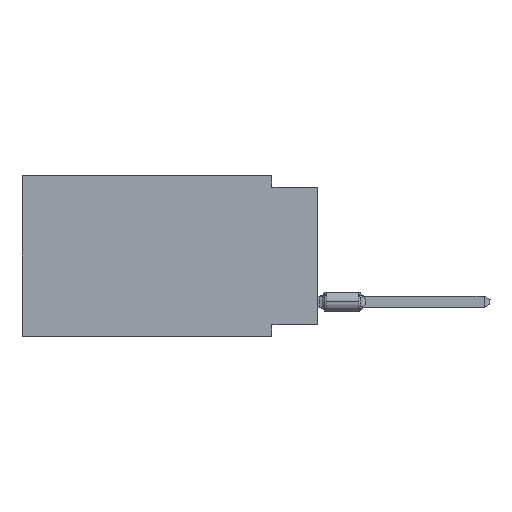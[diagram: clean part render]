
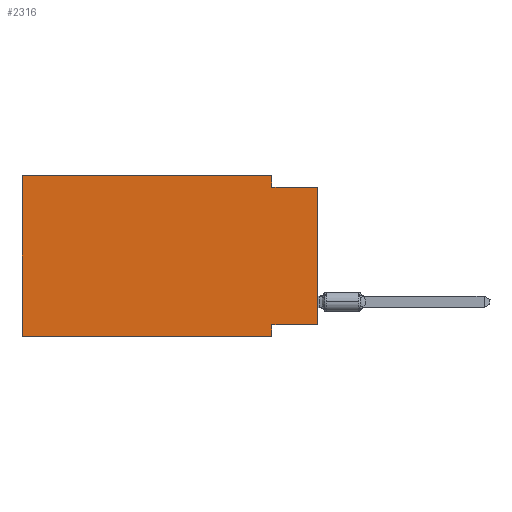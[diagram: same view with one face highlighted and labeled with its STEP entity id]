
A CAD part, left-side view. The second image highlights one B-rep face of the part: STEP entity #2316.
In plain terms, the highlighted planar face has unit normal (-1, 0, 0).
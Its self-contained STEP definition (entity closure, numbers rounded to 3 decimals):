
#332 = DIRECTION ( 'NONE',  ( 0., 0., -1. ) ) ;
#516 = ORIENTED_EDGE ( 'NONE', *, *, #9093, .F. ) ;
#628 = AXIS2_PLACEMENT_3D ( 'NONE', #17649, #9666, #20315 ) ;
#1312 = CARTESIAN_POINT ( 'NONE',  ( 0., 0., -8.255 ) ) ;
#1315 = VERTEX_POINT ( 'NONE', #6627 ) ;
#1503 = ORIENTED_EDGE ( 'NONE', *, *, #3135, .F. ) ;
#1546 = VERTEX_POINT ( 'NONE', #4777 ) ;
#2316 = ADVANCED_FACE ( 'NONE', ( #14979 ), #32851, .F. ) ;
#2844 = LINE ( 'NONE', #13030, #29243 ) ;
#3135 = EDGE_CURVE ( 'NONE', #19617, #12012, #27275, .T. ) ;
#3253 = CARTESIAN_POINT ( 'NONE',  ( 0., 0., 0. ) ) ;
#3286 = LINE ( 'NONE', #28986, #11130 ) ;
#3433 = CARTESIAN_POINT ( 'NONE',  ( 0., 16.383, -8.89 ) ) ;
#4777 = CARTESIAN_POINT ( 'NONE',  ( 0., 0., -0.635 ) ) ;
#5766 = CARTESIAN_POINT ( 'NONE',  ( 0., 2.54, 0. ) ) ;
#6627 = CARTESIAN_POINT ( 'NONE',  ( 0., 2.54, -8.89 ) ) ;
#7154 = ORIENTED_EDGE ( 'NONE', *, *, #18124, .T. ) ;
#7588 = DIRECTION ( 'NONE',  ( 0., -1., 0. ) ) ;
#8592 = DIRECTION ( 'NONE',  ( 0., 0., 1. ) ) ;
#8926 = CARTESIAN_POINT ( 'NONE',  ( 0., 2.54, 0. ) ) ;
#9093 = EDGE_CURVE ( 'NONE', #12012, #32319, #18448, .T. ) ;
#9666 = DIRECTION ( 'NONE',  ( 1., 0., 0. ) ) ;
#9780 = CARTESIAN_POINT ( 'NONE',  ( 0., 16.383, -8.89 ) ) ;
#11091 = VECTOR ( 'NONE', #24778, 1000. ) ;
#11130 = VECTOR ( 'NONE', #31485, 1000. ) ;
#11513 = CARTESIAN_POINT ( 'NONE',  ( 0., 2.54, -0.635 ) ) ;
#11792 = DIRECTION ( 'NONE',  ( 0., -1., 0. ) ) ;
#11896 = CARTESIAN_POINT ( 'NONE',  ( 0., 16.383, 0. ) ) ;
#12012 = VERTEX_POINT ( 'NONE', #8926 ) ;
#12126 = CARTESIAN_POINT ( 'NONE',  ( 0., 0., -0.635 ) ) ;
#12962 = EDGE_CURVE ( 'NONE', #21181, #1315, #2844, .T. ) ;
#13030 = CARTESIAN_POINT ( 'NONE',  ( 0., 2.54, -8.89 ) ) ;
#13249 = ORIENTED_EDGE ( 'NONE', *, *, #13583, .F. ) ;
#13583 = EDGE_CURVE ( 'NONE', #15958, #19617, #3286, .T. ) ;
#13775 = EDGE_CURVE ( 'NONE', #32319, #1546, #17126, .T. ) ;
#14280 = VERTEX_POINT ( 'NONE', #1312 ) ;
#14307 = ORIENTED_EDGE ( 'NONE', *, *, #29996, .T. ) ;
#14979 = FACE_OUTER_BOUND ( 'NONE', #22821, .T. ) ;
#15958 = VERTEX_POINT ( 'NONE', #3433 ) ;
#16891 = DIRECTION ( 'NONE',  ( 0., 1., 0. ) ) ;
#17126 = LINE ( 'NONE', #12126, #19166 ) ;
#17417 = VECTOR ( 'NONE', #31130, 1000. ) ;
#17649 = CARTESIAN_POINT ( 'NONE',  ( 0., 16.383, 0. ) ) ;
#18124 = EDGE_CURVE ( 'NONE', #15958, #1315, #32644, .T. ) ;
#18448 = LINE ( 'NONE', #5766, #17417 ) ;
#18483 = VECTOR ( 'NONE', #8592, 1000. ) ;
#19166 = VECTOR ( 'NONE', #11792, 1000. ) ;
#19617 = VERTEX_POINT ( 'NONE', #11896 ) ;
#20315 = DIRECTION ( 'NONE',  ( 0., 0., -1. ) ) ;
#21181 = VERTEX_POINT ( 'NONE', #21706 ) ;
#21706 = CARTESIAN_POINT ( 'NONE',  ( 0., 2.54, -8.255 ) ) ;
#21956 = ORIENTED_EDGE ( 'NONE', *, *, #13775, .F. ) ;
#22438 = CARTESIAN_POINT ( 'NONE',  ( 0., 16.383, 0. ) ) ;
#22821 = EDGE_LOOP ( 'NONE', ( #14307, #21956, #516, #1503, #13249, #7154, #32328, #29013 ) ) ;
#23015 = VECTOR ( 'NONE', #7588, 1000. ) ;
#24778 = DIRECTION ( 'NONE',  ( 0., -1., 0. ) ) ;
#26124 = LINE ( 'NONE', #3253, #18483 ) ;
#27275 = LINE ( 'NONE', #22438, #11091 ) ;
#28986 = CARTESIAN_POINT ( 'NONE',  ( 0., 16.383, 0. ) ) ;
#29013 = ORIENTED_EDGE ( 'NONE', *, *, #31929, .F. ) ;
#29243 = VECTOR ( 'NONE', #332, 1000. ) ;
#29454 = VECTOR ( 'NONE', #16891, 1000. ) ;
#29996 = EDGE_CURVE ( 'NONE', #14280, #1546, #26124, .T. ) ;
#31130 = DIRECTION ( 'NONE',  ( 0., 0., -1. ) ) ;
#31420 = LINE ( 'NONE', #31748, #29454 ) ;
#31485 = DIRECTION ( 'NONE',  ( 0., 0., 1. ) ) ;
#31748 = CARTESIAN_POINT ( 'NONE',  ( 0., 0., -8.255 ) ) ;
#31929 = EDGE_CURVE ( 'NONE', #14280, #21181, #31420, .T. ) ;
#32319 = VERTEX_POINT ( 'NONE', #11513 ) ;
#32328 = ORIENTED_EDGE ( 'NONE', *, *, #12962, .F. ) ;
#32644 = LINE ( 'NONE', #9780, #23015 ) ;
#32851 = PLANE ( 'NONE',  #628 ) ;
